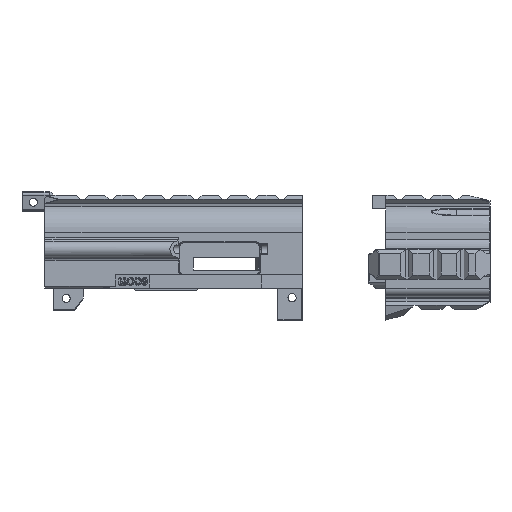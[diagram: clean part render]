
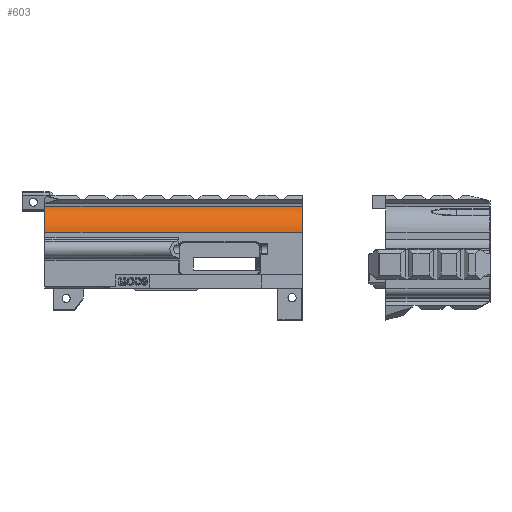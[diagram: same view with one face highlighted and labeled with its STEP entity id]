
A CAD part, top view. The second image highlights one B-rep face of the part: STEP entity #603.
In plain terms, the highlighted cylindrical face has radius 20.1 mm (diameter 40.2 mm), a partial arc.
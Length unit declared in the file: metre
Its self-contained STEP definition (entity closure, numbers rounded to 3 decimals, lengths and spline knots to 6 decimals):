
#603=ADVANCED_FACE('0:10848',(#2448),#2449,.T.);
#2448=FACE_OUTER_BOUND('',#6328,.T.);
#2449=CYLINDRICAL_SURFACE('',#6329,0.0201);
#6328=EDGE_LOOP('',(#13044,#13045,#13046,#13047));
#6329=AXIS2_PLACEMENT_3D('',#13048,#13049,#13050);
#13044=ORIENTED_EDGE('',*,*,#21766,.T.);
#13045=ORIENTED_EDGE('',*,*,#21768,.T.);
#13046=ORIENTED_EDGE('',*,*,#21769,.F.);
#13047=ORIENTED_EDGE('',*,*,#21770,.T.);
#13048=CARTESIAN_POINT('',(-0.020072,0.047361,0.001));
#13049=DIRECTION('',(1.0,0.,0.));
#13050=DIRECTION('',(0.,0.,-1.0));
#21766=EDGE_CURVE('0:13803',#26518,#26516,#26519,.T.);
#21768=EDGE_CURVE('0:13239',#26516,#26521,#26522,.T.);
#21769=EDGE_CURVE('0:13800',#26523,#26521,#26524,.T.);
#21770=EDGE_CURVE('0:13572',#26523,#26518,#26525,.T.);
#26516=VERTEX_POINT('',#35665);
#26518=VERTEX_POINT('',#35668);
#26519=LINE('',#35669,#35670);
#26521=VERTEX_POINT('',#35673);
#26522=CIRCLE('',#35674,0.0201);
#26523=VERTEX_POINT('',#35675);
#26524=LINE('',#35676,#35677);
#26525=CIRCLE('',#35678,0.0201);
#35665=CARTESIAN_POINT('',(-0.178704,0.065991,0.008545));
#35668=CARTESIAN_POINT('',(0.011678,0.065991,0.008545));
#35669=CARTESIAN_POINT('',(-0.020072,0.065991,0.008545));
#35670=VECTOR('',#44561,0.190382);
#35673=CARTESIAN_POINT('',(-0.178704,0.047361,0.0211));
#35674=AXIS2_PLACEMENT_3D('',#44563,#44564,#44565);
#35675=CARTESIAN_POINT('',(0.011678,0.047361,0.0211));
#35676=CARTESIAN_POINT('',(-0.020072,0.047361,0.0211));
#35677=VECTOR('',#44566,0.190382);
#35678=AXIS2_PLACEMENT_3D('',#44567,#44568,#44569);
#44561=DIRECTION('',(-1.0,0.0,0.));
#44563=CARTESIAN_POINT('',(-0.178704,0.047361,0.001));
#44564=DIRECTION('',(1.0,0.,0.));
#44565=DIRECTION('',(0.,0.,-1.0));
#44566=DIRECTION('',(-1.0,0.0,0.));
#44567=CARTESIAN_POINT('',(0.011678,0.047361,0.001));
#44568=DIRECTION('',(-1.0,0.,0.));
#44569=DIRECTION('',(0.,0.,-1.0));
